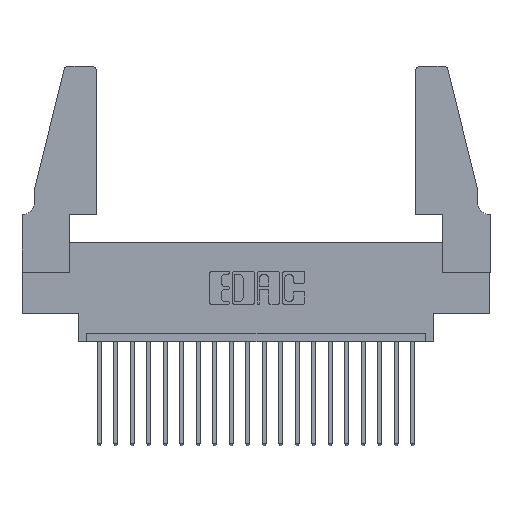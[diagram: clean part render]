
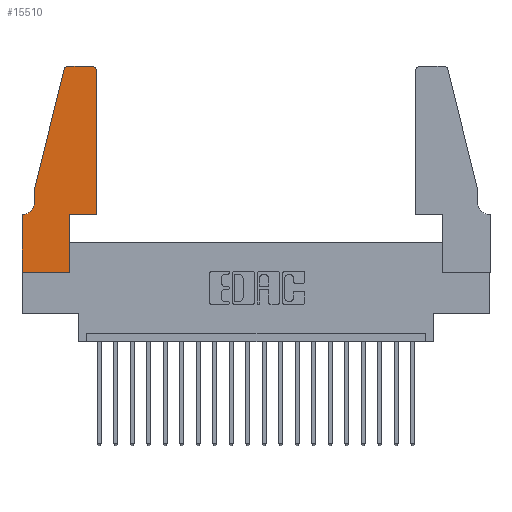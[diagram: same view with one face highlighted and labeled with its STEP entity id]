
A CAD part, top view. The second image highlights one B-rep face of the part: STEP entity #15510.
In plain terms, the highlighted planar face has unit normal (0, 0, 1).
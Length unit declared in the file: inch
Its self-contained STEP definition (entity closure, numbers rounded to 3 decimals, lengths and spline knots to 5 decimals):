
#42 = EDGE_CURVE ( 'NONE', #10576, #8940, #8518, .T. ) ;
#315 = CARTESIAN_POINT ( 'NONE',  ( 0.4505, 0.35, 0.37 ) ) ;
#509 = VERTEX_POINT ( 'NONE', #3327 ) ;
#783 = EDGE_CURVE ( 'NONE', #5313, #10390, #11928, .T. ) ;
#1142 = ORIENTED_EDGE ( 'NONE', *, *, #3537, .T. ) ;
#1472 = VECTOR ( 'NONE', #1966, 39.37008 ) ;
#1589 = AXIS2_PLACEMENT_3D ( 'NONE', #10591, #1766, #2358 ) ;
#1766 = DIRECTION ( 'NONE',  ( 0., 0., 1. ) ) ;
#1934 = CARTESIAN_POINT ( 'NONE',  ( 0.2865, 0.35, 0.37 ) ) ;
#1966 = DIRECTION ( 'NONE',  ( 0., -1., 0. ) ) ;
#2287 = VERTEX_POINT ( 'NONE', #13173 ) ;
#2358 = DIRECTION ( 'NONE',  ( 1., 0., 0. ) ) ;
#2522 = VECTOR ( 'NONE', #12516, 39.37008 ) ;
#2788 = CARTESIAN_POINT ( 'NONE',  ( 0.4505, 0.35, 0.37 ) ) ;
#2967 = FACE_OUTER_BOUND ( 'NONE', #8370, .T. ) ;
#3019 = CARTESIAN_POINT ( 'NONE',  ( 0.0755, 0.42, 0.37 ) ) ;
#3237 = VECTOR ( 'NONE', #9657, 39.37008 ) ;
#3327 = CARTESIAN_POINT ( 'NONE',  ( 0., 0., 0.37 ) ) ;
#3335 = ORIENTED_EDGE ( 'NONE', *, *, #7939, .T. ) ;
#3482 = ORIENTED_EDGE ( 'NONE', *, *, #15358, .T. ) ;
#3537 = EDGE_CURVE ( 'NONE', #8359, #509, #13306, .T. ) ;
#3563 = VECTOR ( 'NONE', #18371, 39.37008 ) ;
#5147 = EDGE_CURVE ( 'NONE', #5817, #11125, #16160, .T. ) ;
#5202 = ORIENTED_EDGE ( 'NONE', *, *, #42, .T. ) ;
#5313 = VERTEX_POINT ( 'NONE', #6468 ) ;
#5453 = VERTEX_POINT ( 'NONE', #9856 ) ;
#5606 = ORIENTED_EDGE ( 'NONE', *, *, #5147, .T. ) ;
#5701 = AXIS2_PLACEMENT_3D ( 'NONE', #15343, #5949, #10666 ) ;
#5817 = VERTEX_POINT ( 'NONE', #14105 ) ;
#5949 = DIRECTION ( 'NONE',  ( 0., 0., 1. ) ) ;
#6468 = CARTESIAN_POINT ( 'NONE',  ( 0.0755, 0.5, 0.37 ) ) ;
#6494 = LINE ( 'NONE', #7640, #2522 ) ;
#6610 = DIRECTION ( 'NONE',  ( 0., 1., 0. ) ) ;
#6620 = CARTESIAN_POINT ( 'NONE',  ( 0.2865, 0., 0.37 ) ) ;
#6966 = VERTEX_POINT ( 'NONE', #17501 ) ;
#7120 = CARTESIAN_POINT ( 'NONE',  ( 0.0755, 0.35, 0.37 ) ) ;
#7289 = CARTESIAN_POINT ( 'NONE',  ( 0.4205, 1.25, 0.37 ) ) ;
#7405 = CARTESIAN_POINT ( 'NONE',  ( 0.2605, 1.25, 0.37 ) ) ;
#7513 = LINE ( 'NONE', #2788, #12682 ) ;
#7562 = AXIS2_PLACEMENT_3D ( 'NONE', #11384, #19305, #19085 ) ;
#7640 = CARTESIAN_POINT ( 'NONE',  ( 0., 0., 0.37 ) ) ;
#7731 = VECTOR ( 'NONE', #15747, 39.37008 ) ;
#7939 = EDGE_CURVE ( 'NONE', #8940, #5817, #7513, .T. ) ;
#7982 = CIRCLE ( 'NONE', #7562, 0.07 ) ;
#8024 = EDGE_CURVE ( 'NONE', #11125, #18784, #20020, .T. ) ;
#8038 = DIRECTION ( 'NONE',  ( 0., 1., 0. ) ) ;
#8042 = CARTESIAN_POINT ( 'NONE',  ( 0.4505, 1.22, 0.37 ) ) ;
#8306 = EDGE_CURVE ( 'NONE', #10390, #5453, #7982, .T. ) ;
#8359 = VERTEX_POINT ( 'NONE', #13224 ) ;
#8370 = EDGE_LOOP ( 'NONE', ( #19370, #17280, #18332, #14207, #17921, #3482, #1142, #19519, #5202, #3335, #5606, #12886 ) ) ;
#8518 = LINE ( 'NONE', #1934, #15621 ) ;
#8940 = VERTEX_POINT ( 'NONE', #14615 ) ;
#8951 = LINE ( 'NONE', #17590, #3237 ) ;
#9657 = DIRECTION ( 'NONE',  ( -0.239, -0.971, 0. ) ) ;
#9670 = LINE ( 'NONE', #7120, #14076 ) ;
#9856 = CARTESIAN_POINT ( 'NONE',  ( 0.0055, 0.35, 0.37 ) ) ;
#10390 = VERTEX_POINT ( 'NONE', #3019 ) ;
#10576 = VERTEX_POINT ( 'NONE', #6620 ) ;
#10591 = CARTESIAN_POINT ( 'NONE',  ( 0.284, 1.22, 0.37 ) ) ;
#10666 = DIRECTION ( 'NONE',  ( 1., 0., 0. ) ) ;
#10850 = DIRECTION ( 'NONE',  ( 0., 0., 1. ) ) ;
#11125 = VERTEX_POINT ( 'NONE', #8042 ) ;
#11384 = CARTESIAN_POINT ( 'NONE',  ( 0.0055, 0.42, 0.37 ) ) ;
#11633 = CIRCLE ( 'NONE', #1589, 0.03 ) ;
#11928 = LINE ( 'NONE', #15881, #7731 ) ;
#12303 = DIRECTION ( 'NONE',  ( 1., 0., 0. ) ) ;
#12401 = DIRECTION ( 'NONE',  ( 1., 0., 0. ) ) ;
#12516 = DIRECTION ( 'NONE',  ( 1., 0., 0. ) ) ;
#12682 = VECTOR ( 'NONE', #12303, 39.37008 ) ;
#12886 = ORIENTED_EDGE ( 'NONE', *, *, #8024, .T. ) ;
#12908 = CARTESIAN_POINT ( 'NONE',  ( 0., 0., 0.37 ) ) ;
#13173 = CARTESIAN_POINT ( 'NONE',  ( 0.284, 1.25, 0.37 ) ) ;
#13224 = CARTESIAN_POINT ( 'NONE',  ( 0., 0.35, 0.37 ) ) ;
#13306 = LINE ( 'NONE', #12908, #1472 ) ;
#13449 = EDGE_CURVE ( 'NONE', #18784, #2287, #13666, .T. ) ;
#13666 = LINE ( 'NONE', #7405, #3563 ) ;
#14076 = VECTOR ( 'NONE', #14804, 39.37008 ) ;
#14105 = CARTESIAN_POINT ( 'NONE',  ( 0.4505, 0.35, 0.37 ) ) ;
#14207 = ORIENTED_EDGE ( 'NONE', *, *, #783, .T. ) ;
#14570 = EDGE_CURVE ( 'NONE', #509, #10576, #6494, .T. ) ;
#14615 = CARTESIAN_POINT ( 'NONE',  ( 0.2865, 0.35, 0.37 ) ) ;
#14617 = AXIS2_PLACEMENT_3D ( 'NONE', #15543, #10850, #12401 ) ;
#14804 = DIRECTION ( 'NONE',  ( -1., 0., 0. ) ) ;
#15343 = CARTESIAN_POINT ( 'NONE',  ( 0.4205, 1.22, 0.37 ) ) ;
#15358 = EDGE_CURVE ( 'NONE', #5453, #8359, #9670, .T. ) ;
#15510 = ADVANCED_FACE ( 'NONE', ( #2967 ), #18627, .T. ) ;
#15543 = CARTESIAN_POINT ( 'NONE',  ( 0., 0.35, 0.37 ) ) ;
#15621 = VECTOR ( 'NONE', #6610, 39.37008 ) ;
#15747 = DIRECTION ( 'NONE',  ( 0., -1., 0. ) ) ;
#15780 = EDGE_CURVE ( 'NONE', #2287, #6966, #11633, .T. ) ;
#15881 = CARTESIAN_POINT ( 'NONE',  ( 0.0755, 0.5, 0.37 ) ) ;
#16160 = LINE ( 'NONE', #315, #18608 ) ;
#17280 = ORIENTED_EDGE ( 'NONE', *, *, #15780, .T. ) ;
#17501 = CARTESIAN_POINT ( 'NONE',  ( 0.25487, 1.22718, 0.37 ) ) ;
#17590 = CARTESIAN_POINT ( 'NONE',  ( 0.0755, 0.5, 0.37 ) ) ;
#17921 = ORIENTED_EDGE ( 'NONE', *, *, #8306, .T. ) ;
#18332 = ORIENTED_EDGE ( 'NONE', *, *, #20169, .T. ) ;
#18371 = DIRECTION ( 'NONE',  ( -1., 0., 0. ) ) ;
#18608 = VECTOR ( 'NONE', #8038, 39.37008 ) ;
#18627 = PLANE ( 'NONE',  #14617 ) ;
#18784 = VERTEX_POINT ( 'NONE', #7289 ) ;
#19085 = DIRECTION ( 'NONE',  ( -1., 0., 0. ) ) ;
#19305 = DIRECTION ( 'NONE',  ( 0., 0., -1. ) ) ;
#19370 = ORIENTED_EDGE ( 'NONE', *, *, #13449, .T. ) ;
#19519 = ORIENTED_EDGE ( 'NONE', *, *, #14570, .T. ) ;
#20020 = CIRCLE ( 'NONE', #5701, 0.03 ) ;
#20169 = EDGE_CURVE ( 'NONE', #6966, #5313, #8951, .T. ) ;
